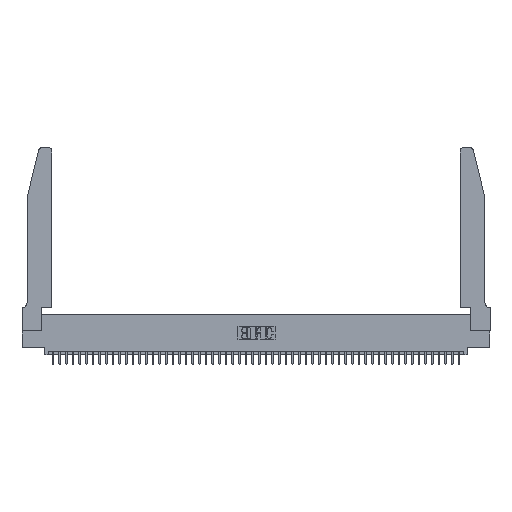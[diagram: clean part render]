
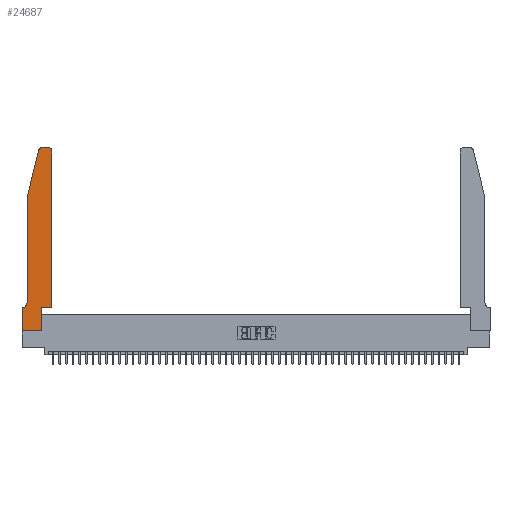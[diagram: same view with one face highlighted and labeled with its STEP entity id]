
A CAD part, top view. The second image highlights one B-rep face of the part: STEP entity #24687.
In plain terms, the highlighted planar face has unit normal (0, 0, 1).
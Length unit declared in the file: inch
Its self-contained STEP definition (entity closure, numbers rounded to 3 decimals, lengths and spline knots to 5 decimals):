
#1070 = EDGE_CURVE ( 'NONE', #15860, #7689, #7773, .T. ) ;
#1272 = DIRECTION ( 'NONE',  ( 0., 0., 1. ) ) ;
#1446 = EDGE_CURVE ( 'NONE', #20762, #6424, #23108, .T. ) ;
#1617 = EDGE_CURVE ( 'NONE', #38602, #23371, #7721, .T. ) ;
#1892 = AXIS2_PLACEMENT_3D ( 'NONE', #22803, #26923, #3316 ) ;
#2176 = CARTESIAN_POINT ( 'NONE',  ( 0.0055, 0.35, 0.37 ) ) ;
#3032 = DIRECTION ( 'NONE',  ( -1., 0., 0. ) ) ;
#3093 = CARTESIAN_POINT ( 'NONE',  ( 0.284, 2.75, 0.37 ) ) ;
#3316 = DIRECTION ( 'NONE',  ( 1., 0., 0. ) ) ;
#4369 = VECTOR ( 'NONE', #42792, 39.37008 ) ;
#4497 = DIRECTION ( 'NONE',  ( 0., -1., 0. ) ) ;
#5470 = CARTESIAN_POINT ( 'NONE',  ( 0.0755, 2., 0.37 ) ) ;
#5768 = DIRECTION ( 'NONE',  ( 0., 0., 1. ) ) ;
#5781 = CARTESIAN_POINT ( 'NONE',  ( 0.2865, 0.35, 0.37 ) ) ;
#6424 = VERTEX_POINT ( 'NONE', #5470 ) ;
#7178 = LINE ( 'NONE', #39769, #37326 ) ;
#7689 = VERTEX_POINT ( 'NONE', #47733 ) ;
#7721 = LINE ( 'NONE', #20955, #35393 ) ;
#7773 = LINE ( 'NONE', #36614, #39149 ) ;
#8835 = ORIENTED_EDGE ( 'NONE', *, *, #1070, .T. ) ;
#9320 = EDGE_CURVE ( 'NONE', #24178, #50598, #50104, .T. ) ;
#9524 = DIRECTION ( 'NONE',  ( 1., 0., 0. ) ) ;
#11527 = VERTEX_POINT ( 'NONE', #18505 ) ;
#11797 = VECTOR ( 'NONE', #45827, 39.37008 ) ;
#12089 = ORIENTED_EDGE ( 'NONE', *, *, #27167, .T. ) ;
#12647 = VECTOR ( 'NONE', #46647, 39.37008 ) ;
#13064 = DIRECTION ( 'NONE',  ( -1., 0., 0. ) ) ;
#13137 = CIRCLE ( 'NONE', #13195, 0.03 ) ;
#13195 = AXIS2_PLACEMENT_3D ( 'NONE', #24905, #1272, #28869 ) ;
#13338 = EDGE_CURVE ( 'NONE', #11527, #24178, #24573, .T. ) ;
#13625 = ORIENTED_EDGE ( 'NONE', *, *, #13338, .T. ) ;
#14604 = EDGE_CURVE ( 'NONE', #23371, #20762, #40500, .T. ) ;
#15860 = VERTEX_POINT ( 'NONE', #2176 ) ;
#17211 = ORIENTED_EDGE ( 'NONE', *, *, #45828, .T. ) ;
#17996 = ORIENTED_EDGE ( 'NONE', *, *, #9320, .T. ) ;
#18377 = CARTESIAN_POINT ( 'NONE',  ( 0.4505, 0.35, 0.37 ) ) ;
#18505 = CARTESIAN_POINT ( 'NONE',  ( 0.2865, 0., 0.37 ) ) ;
#18614 = ORIENTED_EDGE ( 'NONE', *, *, #1446, .T. ) ;
#19293 = VERTEX_POINT ( 'NONE', #40953 ) ;
#19407 = CARTESIAN_POINT ( 'NONE',  ( 0.0755, 2., 0.37 ) ) ;
#19611 = VERTEX_POINT ( 'NONE', #27334 ) ;
#19664 = EDGE_LOOP ( 'NONE', ( #27678, #27841, #18614, #12089, #34838, #8835, #17211, #42203, #13625, #17996, #29807, #21851 ) ) ;
#20762 = VERTEX_POINT ( 'NONE', #30001 ) ;
#20955 = CARTESIAN_POINT ( 'NONE',  ( 0.2605, 2.75, 0.37 ) ) ;
#21851 = ORIENTED_EDGE ( 'NONE', *, *, #41208, .T. ) ;
#22502 = FACE_OUTER_BOUND ( 'NONE', #19664, .T. ) ;
#22529 = VECTOR ( 'NONE', #9524, 39.37008 ) ;
#22803 = CARTESIAN_POINT ( 'NONE',  ( 0., 0.35, 0.37 ) ) ;
#23108 = LINE ( 'NONE', #42743, #12647 ) ;
#23371 = VERTEX_POINT ( 'NONE', #3093 ) ;
#24178 = VERTEX_POINT ( 'NONE', #27842 ) ;
#24573 = LINE ( 'NONE', #5781, #35013 ) ;
#24687 = ADVANCED_FACE ( 'NONE', ( #22502 ), #50371, .T. ) ;
#24897 = DIRECTION ( 'NONE',  ( -1., 0., 0. ) ) ;
#24905 = CARTESIAN_POINT ( 'NONE',  ( 0.4205, 2.72, 0.37 ) ) ;
#25394 = DIRECTION ( 'NONE',  ( 0., 1., 0. ) ) ;
#26430 = VERTEX_POINT ( 'NONE', #49501 ) ;
#26630 = DIRECTION ( 'NONE',  ( 0., 0., -1. ) ) ;
#26923 = DIRECTION ( 'NONE',  ( 0., 0., 1. ) ) ;
#27167 = EDGE_CURVE ( 'NONE', #6424, #19293, #43723, .T. ) ;
#27334 = CARTESIAN_POINT ( 'NONE',  ( 0., 0., 0.37 ) ) ;
#27678 = ORIENTED_EDGE ( 'NONE', *, *, #1617, .T. ) ;
#27841 = ORIENTED_EDGE ( 'NONE', *, *, #14604, .T. ) ;
#27842 = CARTESIAN_POINT ( 'NONE',  ( 0.2865, 0.35, 0.37 ) ) ;
#28869 = DIRECTION ( 'NONE',  ( 1., 0., 0. ) ) ;
#29332 = CARTESIAN_POINT ( 'NONE',  ( 0.284, 2.72, 0.37 ) ) ;
#29807 = ORIENTED_EDGE ( 'NONE', *, *, #30847, .T. ) ;
#30001 = CARTESIAN_POINT ( 'NONE',  ( 0.25487, 2.72718, 0.37 ) ) ;
#30847 = EDGE_CURVE ( 'NONE', #50598, #26430, #35791, .T. ) ;
#33085 = CARTESIAN_POINT ( 'NONE',  ( 0.4505, 0.35, 0.37 ) ) ;
#33261 = DIRECTION ( 'NONE',  ( 1., 0., 0. ) ) ;
#33814 = CARTESIAN_POINT ( 'NONE',  ( 0., 0., 0.37 ) ) ;
#34116 = CIRCLE ( 'NONE', #48944, 0.07 ) ;
#34838 = ORIENTED_EDGE ( 'NONE', *, *, #39084, .T. ) ;
#35013 = VECTOR ( 'NONE', #25394, 39.37008 ) ;
#35393 = VECTOR ( 'NONE', #24897, 39.37008 ) ;
#35791 = LINE ( 'NONE', #18377, #11797 ) ;
#36614 = CARTESIAN_POINT ( 'NONE',  ( 0.0755, 0.35, 0.37 ) ) ;
#37326 = VECTOR ( 'NONE', #4497, 39.37008 ) ;
#38602 = VERTEX_POINT ( 'NONE', #47224 ) ;
#39084 = EDGE_CURVE ( 'NONE', #19293, #15860, #34116, .T. ) ;
#39149 = VECTOR ( 'NONE', #13064, 39.37008 ) ;
#39769 = CARTESIAN_POINT ( 'NONE',  ( 0., 0., 0.37 ) ) ;
#40500 = CIRCLE ( 'NONE', #43494, 0.03 ) ;
#40953 = CARTESIAN_POINT ( 'NONE',  ( 0.0755, 0.42, 0.37 ) ) ;
#41208 = EDGE_CURVE ( 'NONE', #26430, #38602, #13137, .T. ) ;
#42203 = ORIENTED_EDGE ( 'NONE', *, *, #43339, .T. ) ;
#42743 = CARTESIAN_POINT ( 'NONE',  ( 0.0755, 2., 0.37 ) ) ;
#42792 = DIRECTION ( 'NONE',  ( 0., -1., 0. ) ) ;
#43339 = EDGE_CURVE ( 'NONE', #19611, #11527, #47352, .T. ) ;
#43494 = AXIS2_PLACEMENT_3D ( 'NONE', #29332, #5768, #33261 ) ;
#43723 = LINE ( 'NONE', #19407, #4369 ) ;
#44863 = CARTESIAN_POINT ( 'NONE',  ( 0.4505, 0.35, 0.37 ) ) ;
#45827 = DIRECTION ( 'NONE',  ( 0., 1., 0. ) ) ;
#45828 = EDGE_CURVE ( 'NONE', #7689, #19611, #7178, .T. ) ;
#46139 = VECTOR ( 'NONE', #49545, 39.37008 ) ;
#46647 = DIRECTION ( 'NONE',  ( -0.239, -0.971, 0. ) ) ;
#47224 = CARTESIAN_POINT ( 'NONE',  ( 0.4205, 2.75, 0.37 ) ) ;
#47352 = LINE ( 'NONE', #33814, #46139 ) ;
#47733 = CARTESIAN_POINT ( 'NONE',  ( 0., 0.35, 0.37 ) ) ;
#48944 = AXIS2_PLACEMENT_3D ( 'NONE', #50087, #26630, #3032 ) ;
#49501 = CARTESIAN_POINT ( 'NONE',  ( 0.4505, 2.72, 0.37 ) ) ;
#49545 = DIRECTION ( 'NONE',  ( 1., 0., 0. ) ) ;
#50087 = CARTESIAN_POINT ( 'NONE',  ( 0.0055, 0.42, 0.37 ) ) ;
#50104 = LINE ( 'NONE', #33085, #22529 ) ;
#50371 = PLANE ( 'NONE',  #1892 ) ;
#50598 = VERTEX_POINT ( 'NONE', #44863 ) ;
